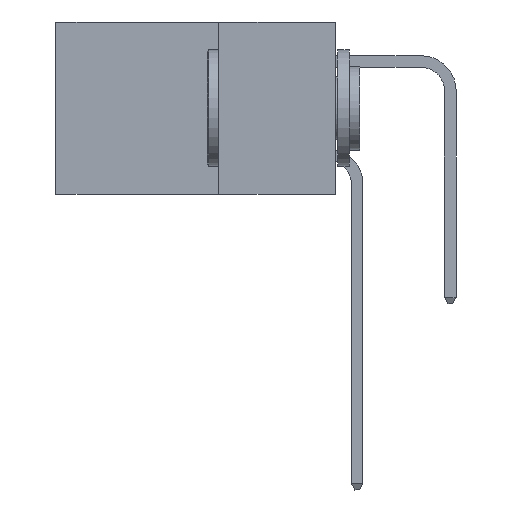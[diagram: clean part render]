
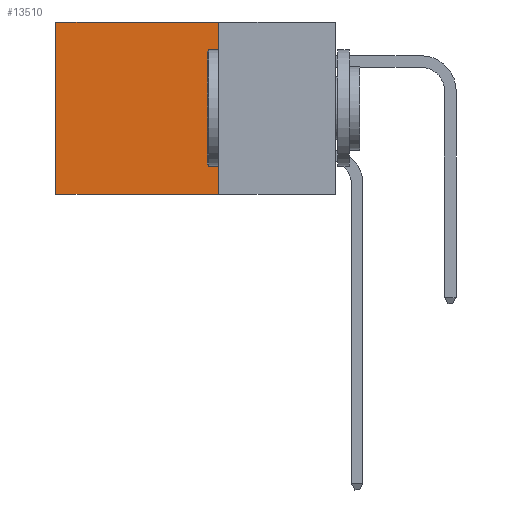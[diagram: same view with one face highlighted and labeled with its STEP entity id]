
A CAD part, left-side view. The second image highlights one B-rep face of the part: STEP entity #13510.
In plain terms, the highlighted planar face has unit normal (-1, 0, 0).
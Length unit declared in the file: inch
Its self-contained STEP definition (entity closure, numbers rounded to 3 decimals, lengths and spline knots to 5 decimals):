
#28 = EDGE_CURVE ( 'NONE', #3485, #12016, #9926, .T. ) ;
#206 = ORIENTED_EDGE ( 'NONE', *, *, #7632, .T. ) ;
#258 = EDGE_CURVE ( 'NONE', #3485, #8873, #8983, .T. ) ;
#828 = ORIENTED_EDGE ( 'NONE', *, *, #28, .F. ) ;
#2041 = CARTESIAN_POINT ( 'NONE',  ( 0.2875, 0.25, 0. ) ) ;
#2457 = VECTOR ( 'NONE', #2940, 39.37008 ) ;
#2940 = DIRECTION ( 'NONE',  ( 0., 1., 0. ) ) ;
#3485 = VERTEX_POINT ( 'NONE', #12321 ) ;
#3903 = CARTESIAN_POINT ( 'NONE',  ( 0.2875, 0.25, -0.37 ) ) ;
#3927 = CARTESIAN_POINT ( 'NONE',  ( 0.2875, 0.25, 0. ) ) ;
#4021 = EDGE_CURVE ( 'NONE', #12016, #10520, #8695, .T. ) ;
#4311 = CARTESIAN_POINT ( 'NONE',  ( 0.2875, 0.6, -0.37 ) ) ;
#4347 = DIRECTION ( 'NONE',  ( 0., 0., -1. ) ) ;
#4374 = VECTOR ( 'NONE', #6102, 39.37008 ) ;
#5243 = EDGE_LOOP ( 'NONE', ( #206, #9696, #828, #10637 ) ) ;
#6075 = DIRECTION ( 'NONE',  ( 0., 0., -1. ) ) ;
#6102 = DIRECTION ( 'NONE',  ( 0., 1., 0. ) ) ;
#6687 = DIRECTION ( 'NONE',  ( 1., 0., 0. ) ) ;
#7632 = EDGE_CURVE ( 'NONE', #8873, #10520, #9286, .T. ) ;
#8101 = CARTESIAN_POINT ( 'NONE',  ( 0.2875, 0.25, -0.37 ) ) ;
#8695 = LINE ( 'NONE', #3903, #2457 ) ;
#8873 = VERTEX_POINT ( 'NONE', #11523 ) ;
#8983 = LINE ( 'NONE', #2041, #4374 ) ;
#9286 = LINE ( 'NONE', #13221, #11435 ) ;
#9696 = ORIENTED_EDGE ( 'NONE', *, *, #4021, .F. ) ;
#9926 = LINE ( 'NONE', #3927, #13362 ) ;
#10269 = PLANE ( 'NONE',  #12619 ) ;
#10520 = VERTEX_POINT ( 'NONE', #4311 ) ;
#10637 = ORIENTED_EDGE ( 'NONE', *, *, #258, .T. ) ;
#11435 = VECTOR ( 'NONE', #13421, 39.37008 ) ;
#11523 = CARTESIAN_POINT ( 'NONE',  ( 0.2875, 0.6, 0. ) ) ;
#11527 = CARTESIAN_POINT ( 'NONE',  ( 0.2875, 0.25, 0. ) ) ;
#12016 = VERTEX_POINT ( 'NONE', #8101 ) ;
#12321 = CARTESIAN_POINT ( 'NONE',  ( 0.2875, 0.25, 0. ) ) ;
#12619 = AXIS2_PLACEMENT_3D ( 'NONE', #11527, #6687, #4347 ) ;
#13104 = FACE_OUTER_BOUND ( 'NONE', #5243, .T. ) ;
#13221 = CARTESIAN_POINT ( 'NONE',  ( 0.2875, 0.6, 0. ) ) ;
#13362 = VECTOR ( 'NONE', #6075, 39.37008 ) ;
#13421 = DIRECTION ( 'NONE',  ( 0., 0., -1. ) ) ;
#13510 = ADVANCED_FACE ( 'NONE', ( #13104 ), #10269, .F. ) ;
